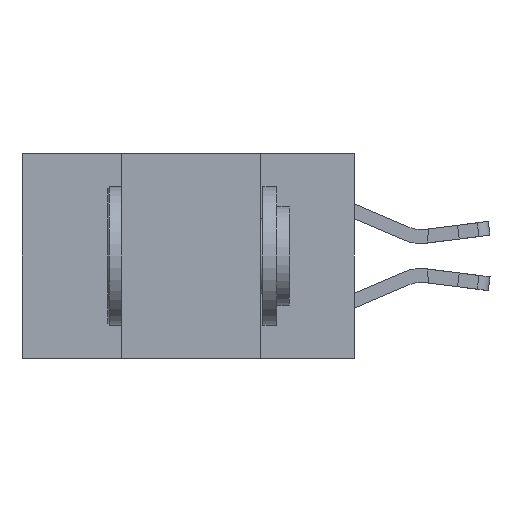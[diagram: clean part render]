
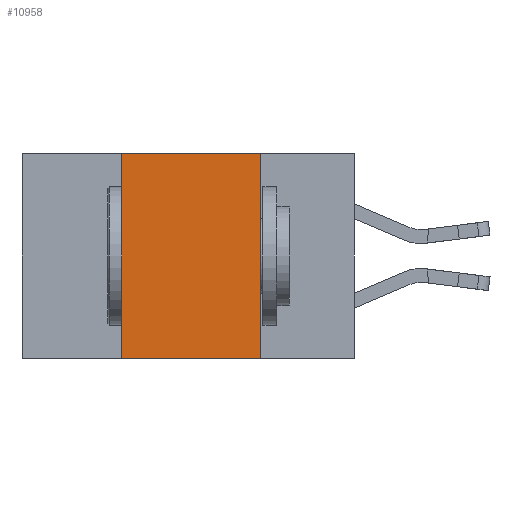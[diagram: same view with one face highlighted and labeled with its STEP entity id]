
A CAD part, left-side view. The second image highlights one B-rep face of the part: STEP entity #10958.
In plain terms, the highlighted planar face has unit normal (-1, 0, 0).
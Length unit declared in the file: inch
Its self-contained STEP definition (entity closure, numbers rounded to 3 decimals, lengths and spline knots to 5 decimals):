
#470 = VECTOR ( 'NONE', #1755, 39.37008 ) ;
#605 = ORIENTED_EDGE ( 'NONE', *, *, #2746, .F. ) ;
#1755 = DIRECTION ( 'NONE',  ( 0., -1., 0. ) ) ;
#2326 = FACE_OUTER_BOUND ( 'NONE', #11248, .T. ) ;
#2441 = CARTESIAN_POINT ( 'NONE',  ( 0., 0.6, 0. ) ) ;
#2537 = CARTESIAN_POINT ( 'NONE',  ( 0., 0.17, -0.37 ) ) ;
#2746 = EDGE_CURVE ( 'NONE', #4583, #6010, #6622, .T. ) ;
#3098 = CARTESIAN_POINT ( 'NONE',  ( 0., 0.17, 0. ) ) ;
#3250 = VECTOR ( 'NONE', #6200, 39.37008 ) ;
#3465 = DIRECTION ( 'NONE',  ( 1., 0., 0. ) ) ;
#3674 = ORIENTED_EDGE ( 'NONE', *, *, #4987, .F. ) ;
#4191 = VERTEX_POINT ( 'NONE', #6930 ) ;
#4583 = VERTEX_POINT ( 'NONE', #3098 ) ;
#4736 = VECTOR ( 'NONE', #10994, 39.37008 ) ;
#4987 = EDGE_CURVE ( 'NONE', #7720, #4583, #9901, .T. ) ;
#5669 = AXIS2_PLACEMENT_3D ( 'NONE', #2441, #3465, #10654 ) ;
#6010 = VERTEX_POINT ( 'NONE', #2537 ) ;
#6200 = DIRECTION ( 'NONE',  ( 0., 0., -1. ) ) ;
#6281 = CARTESIAN_POINT ( 'NONE',  ( 0., 0.17, -0.37 ) ) ;
#6622 = LINE ( 'NONE', #6281, #3250 ) ;
#6930 = CARTESIAN_POINT ( 'NONE',  ( 0., 0.42, -0.37 ) ) ;
#7612 = CARTESIAN_POINT ( 'NONE',  ( 0., 0.42, 0. ) ) ;
#7720 = VERTEX_POINT ( 'NONE', #7612 ) ;
#8712 = LINE ( 'NONE', #12932, #470 ) ;
#9501 = ORIENTED_EDGE ( 'NONE', *, *, #11000, .F. ) ;
#9765 = CARTESIAN_POINT ( 'NONE',  ( 0., 0.6, 0. ) ) ;
#9901 = LINE ( 'NONE', #9765, #4736 ) ;
#9915 = LINE ( 'NONE', #10701, #12259 ) ;
#10654 = DIRECTION ( 'NONE',  ( 0., 0., -1. ) ) ;
#10701 = CARTESIAN_POINT ( 'NONE',  ( 0., 0.42, -0.37 ) ) ;
#10958 = ADVANCED_FACE ( 'NONE', ( #2326 ), #11652, .F. ) ;
#10994 = DIRECTION ( 'NONE',  ( 0., -1., 0. ) ) ;
#11000 = EDGE_CURVE ( 'NONE', #4191, #7720, #9915, .T. ) ;
#11075 = ORIENTED_EDGE ( 'NONE', *, *, #13125, .T. ) ;
#11248 = EDGE_LOOP ( 'NONE', ( #605, #3674, #9501, #11075 ) ) ;
#11652 = PLANE ( 'NONE',  #5669 ) ;
#11731 = DIRECTION ( 'NONE',  ( 0., 0., 1. ) ) ;
#12259 = VECTOR ( 'NONE', #11731, 39.37008 ) ;
#12932 = CARTESIAN_POINT ( 'NONE',  ( 0., 0.6, -0.37 ) ) ;
#13125 = EDGE_CURVE ( 'NONE', #4191, #6010, #8712, .T. ) ;
